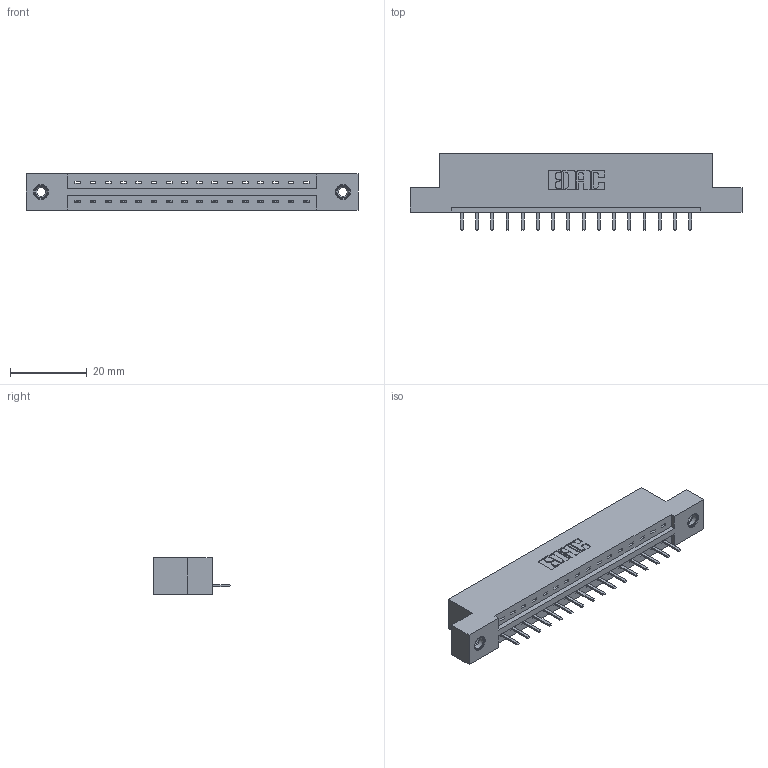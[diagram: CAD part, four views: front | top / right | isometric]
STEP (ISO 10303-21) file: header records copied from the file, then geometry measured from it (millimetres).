
FILE_DESCRIPTION (( 'STEP AP203' ), '1' );
FILE_NAME ('337-016-520-108.STEP', '2018-08-04T18:02:31', ( '' ), ( '' ), 'SwSTEP 2.0', 'SolidWorks 2016', '' );
FILE_SCHEMA (( 'CONFIG_CONTROL_DESIGN' ));
Length unit declared in the file: inch
Products named in the file (4): 337 Part_Flush Mounting Lugs - 0.156 Dia-TI; 345-292-001_345-293-120; 345-250-001_345-250-003-102; 337-016-520-108
Assembly tree (19 placements, depth 2):
  337-016-520-108
    337 Part_Flush Mounting Lugs - 0.156 Dia-TI
    345-292-001_345-293-120  x16
    345-250-001_345-250-003-102  x2
Bounding box: 86.41 x 20.02 x 9.4 mm (x, y, z)
Volume: 8603 mm3; surface area: 8609.7 mm2
Topology: 19 solids, 19 shells, 1230 faces, 3583 edges, 2338 vertices
Faces by surface type: plane 870, cylinder 344, cone 12, torus 4
Entity records: 16556 total; most frequent: CARTESIAN_POINT 2873, ORIENTED_EDGE 2806, DIRECTION 2493, EDGE_CURVE 1403, VECTOR 1251, LINE 1251, VERTEX_POINT 928, AXIS2_PLACEMENT_3D 621
